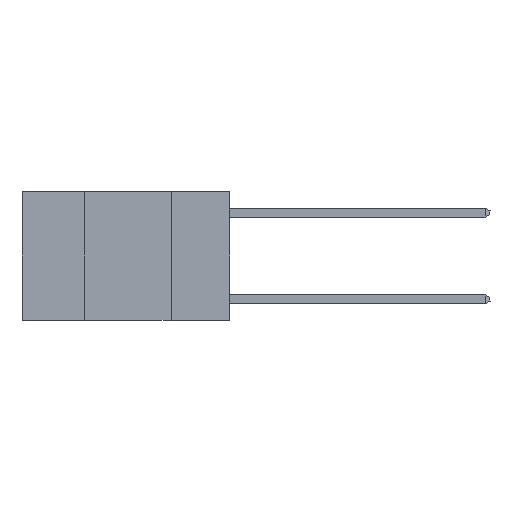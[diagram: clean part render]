
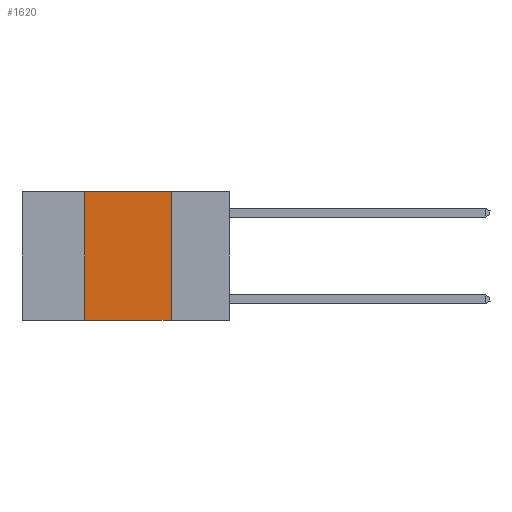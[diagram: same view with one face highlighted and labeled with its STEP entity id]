
A CAD part, left-side view. The second image highlights one B-rep face of the part: STEP entity #1620.
In plain terms, the highlighted planar face has unit normal (-1, 0, 0).
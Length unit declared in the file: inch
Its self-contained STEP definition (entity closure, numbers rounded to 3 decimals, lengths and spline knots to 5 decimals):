
#964 = VERTEX_POINT ( 'NONE', #24241 ) ;
#1620 = ADVANCED_FACE ( 'NONE', ( #25321 ), #3190, .F. ) ;
#2435 = EDGE_CURVE ( 'NONE', #18384, #6434, #9824, .T. ) ;
#3190 = PLANE ( 'NONE',  #7699 ) ;
#3283 = EDGE_LOOP ( 'NONE', ( #9976, #22274, #5469, #14667 ) ) ;
#3316 = CARTESIAN_POINT ( 'NONE',  ( 0., 0.17, 0. ) ) ;
#3327 = CARTESIAN_POINT ( 'NONE',  ( 0., 0.6, 0. ) ) ;
#3687 = CARTESIAN_POINT ( 'NONE',  ( 0., 0.6, -0.37 ) ) ;
#4534 = CARTESIAN_POINT ( 'NONE',  ( 0., 0.17, -0.37 ) ) ;
#4982 = VECTOR ( 'NONE', #12298, 39.37008 ) ;
#5469 = ORIENTED_EDGE ( 'NONE', *, *, #13251, .F. ) ;
#5732 = LINE ( 'NONE', #3687, #23164 ) ;
#6434 = VERTEX_POINT ( 'NONE', #3316 ) ;
#7699 = AXIS2_PLACEMENT_3D ( 'NONE', #3327, #21102, #18906 ) ;
#8412 = DIRECTION ( 'NONE',  ( 0., 0., 1. ) ) ;
#9824 = LINE ( 'NONE', #23070, #4982 ) ;
#9976 = ORIENTED_EDGE ( 'NONE', *, *, #25559, .F. ) ;
#12298 = DIRECTION ( 'NONE',  ( 0., -1., 0. ) ) ;
#12301 = DIRECTION ( 'NONE',  ( 0., -1., 0. ) ) ;
#12804 = VERTEX_POINT ( 'NONE', #4534 ) ;
#13251 = EDGE_CURVE ( 'NONE', #964, #18384, #23840, .T. ) ;
#13710 = VECTOR ( 'NONE', #28704, 39.37008 ) ;
#14667 = ORIENTED_EDGE ( 'NONE', *, *, #15515, .T. ) ;
#15515 = EDGE_CURVE ( 'NONE', #964, #12804, #5732, .T. ) ;
#15742 = LINE ( 'NONE', #22140, #13710 ) ;
#16719 = CARTESIAN_POINT ( 'NONE',  ( 0., 0.42, 0. ) ) ;
#18384 = VERTEX_POINT ( 'NONE', #27105 ) ;
#18906 = DIRECTION ( 'NONE',  ( 0., 0., -1. ) ) ;
#21102 = DIRECTION ( 'NONE',  ( 1., 0., 0. ) ) ;
#22140 = CARTESIAN_POINT ( 'NONE',  ( 0., 0.17, 0. ) ) ;
#22274 = ORIENTED_EDGE ( 'NONE', *, *, #2435, .F. ) ;
#23070 = CARTESIAN_POINT ( 'NONE',  ( 0., 0.6, 0. ) ) ;
#23164 = VECTOR ( 'NONE', #12301, 39.37008 ) ;
#23840 = LINE ( 'NONE', #16719, #23986 ) ;
#23986 = VECTOR ( 'NONE', #8412, 39.37008 ) ;
#24241 = CARTESIAN_POINT ( 'NONE',  ( 0., 0.42, -0.37 ) ) ;
#25321 = FACE_OUTER_BOUND ( 'NONE', #3283, .T. ) ;
#25559 = EDGE_CURVE ( 'NONE', #6434, #12804, #15742, .T. ) ;
#27105 = CARTESIAN_POINT ( 'NONE',  ( 0., 0.42, 0. ) ) ;
#28704 = DIRECTION ( 'NONE',  ( 0., 0., -1. ) ) ;
